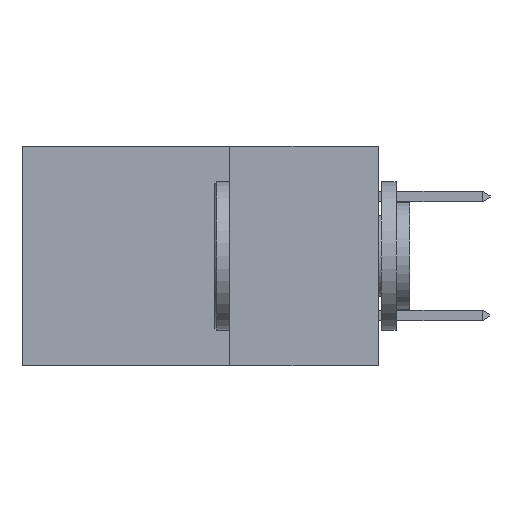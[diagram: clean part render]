
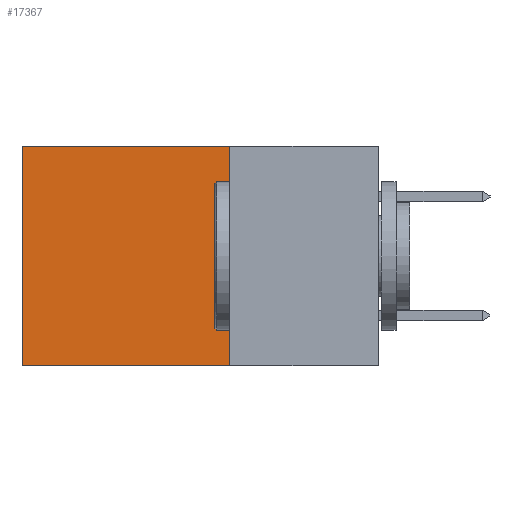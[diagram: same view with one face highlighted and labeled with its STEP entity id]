
A CAD part, left-side view. The second image highlights one B-rep face of the part: STEP entity #17367.
In plain terms, the highlighted planar face has unit normal (-1, 0, 0).
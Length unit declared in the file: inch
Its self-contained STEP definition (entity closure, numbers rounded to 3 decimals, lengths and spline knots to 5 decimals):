
#966 = DIRECTION ( 'NONE',  ( 0., 0., -1. ) ) ;
#1964 = EDGE_CURVE ( 'NONE', #9608, #18667, #12703, .T. ) ;
#2036 = VERTEX_POINT ( 'NONE', #9889 ) ;
#3302 = CARTESIAN_POINT ( 'NONE',  ( 0.298, 0.25, 0. ) ) ;
#4985 = VECTOR ( 'NONE', #6403, 39.37008 ) ;
#6403 = DIRECTION ( 'NONE',  ( 0., 1., 0. ) ) ;
#6562 = VECTOR ( 'NONE', #966, 39.37008 ) ;
#6599 = DIRECTION ( 'NONE',  ( 1., 0., 0. ) ) ;
#6751 = CARTESIAN_POINT ( 'NONE',  ( 0.298, 0.25, 0. ) ) ;
#7215 = CARTESIAN_POINT ( 'NONE',  ( 0.298, 0.25, -0.37 ) ) ;
#8458 = DIRECTION ( 'NONE',  ( 0., 0., -1. ) ) ;
#9111 = FACE_OUTER_BOUND ( 'NONE', #20873, .T. ) ;
#9119 = DIRECTION ( 'NONE',  ( 0., 1., 0. ) ) ;
#9608 = VERTEX_POINT ( 'NONE', #25790 ) ;
#9889 = CARTESIAN_POINT ( 'NONE',  ( 0.298, 0.6, -0.37 ) ) ;
#12136 = CARTESIAN_POINT ( 'NONE',  ( 0.298, 0.6, 0. ) ) ;
#12703 = LINE ( 'NONE', #3302, #6562 ) ;
#13036 = EDGE_CURVE ( 'NONE', #18667, #2036, #29138, .T. ) ;
#14403 = EDGE_CURVE ( 'NONE', #9608, #19447, #29053, .T. ) ;
#14522 = ORIENTED_EDGE ( 'NONE', *, *, #14403, .T. ) ;
#17367 = ADVANCED_FACE ( 'NONE', ( #9111 ), #26992, .F. ) ;
#17769 = VECTOR ( 'NONE', #8458, 39.37008 ) ;
#17858 = CARTESIAN_POINT ( 'NONE',  ( 0.298, 0.25, -0.37 ) ) ;
#18667 = VERTEX_POINT ( 'NONE', #7215 ) ;
#19447 = VERTEX_POINT ( 'NONE', #12136 ) ;
#20364 = CARTESIAN_POINT ( 'NONE',  ( 0.298, 0.25, 0. ) ) ;
#20873 = EDGE_LOOP ( 'NONE', ( #22102, #26577, #22704, #14522 ) ) ;
#22102 = ORIENTED_EDGE ( 'NONE', *, *, #22854, .T. ) ;
#22653 = DIRECTION ( 'NONE',  ( 0., 0., -1. ) ) ;
#22704 = ORIENTED_EDGE ( 'NONE', *, *, #1964, .F. ) ;
#22854 = EDGE_CURVE ( 'NONE', #19447, #2036, #23826, .T. ) ;
#23826 = LINE ( 'NONE', #28723, #17769 ) ;
#25790 = CARTESIAN_POINT ( 'NONE',  ( 0.298, 0.25, 0. ) ) ;
#26577 = ORIENTED_EDGE ( 'NONE', *, *, #13036, .F. ) ;
#26992 = PLANE ( 'NONE',  #29480 ) ;
#27700 = VECTOR ( 'NONE', #9119, 39.37008 ) ;
#28723 = CARTESIAN_POINT ( 'NONE',  ( 0.298, 0.6, 0. ) ) ;
#29053 = LINE ( 'NONE', #6751, #27700 ) ;
#29138 = LINE ( 'NONE', #17858, #4985 ) ;
#29480 = AXIS2_PLACEMENT_3D ( 'NONE', #20364, #6599, #22653 ) ;
